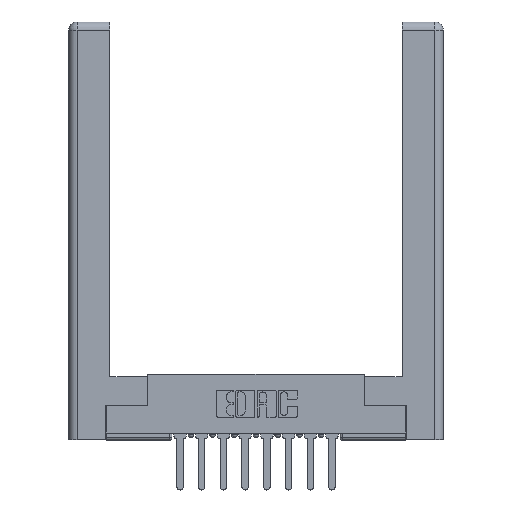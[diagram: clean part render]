
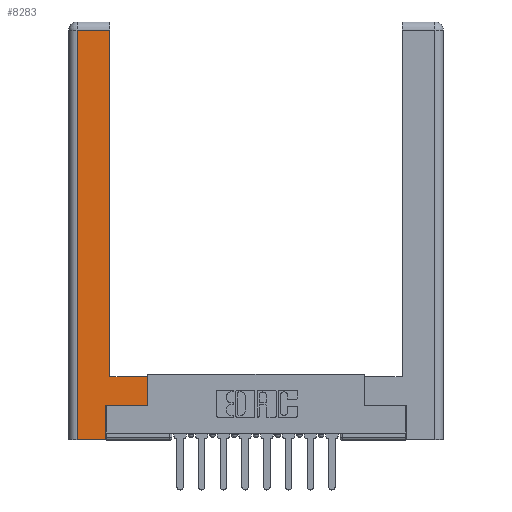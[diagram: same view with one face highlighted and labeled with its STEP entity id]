
A CAD part, top view. The second image highlights one B-rep face of the part: STEP entity #8283.
In plain terms, the highlighted planar face has unit normal (0, 0, 1).
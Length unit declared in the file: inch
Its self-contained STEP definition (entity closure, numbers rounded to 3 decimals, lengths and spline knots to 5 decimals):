
#43 = CARTESIAN_POINT ( 'NONE',  ( 0.295, 2.94, 0. ) ) ;
#262 = CARTESIAN_POINT ( 'NONE',  ( 0.0615, 2.94, 0. ) ) ;
#449 = CARTESIAN_POINT ( 'NONE',  ( 0.265, 0.245, 0. ) ) ;
#627 = VECTOR ( 'NONE', #13145, 39.37008 ) ;
#644 = AXIS2_PLACEMENT_3D ( 'NONE', #8451, #4155, #2939 ) ;
#757 = CARTESIAN_POINT ( 'NONE',  ( 0.565, 0.45, 0. ) ) ;
#957 = CARTESIAN_POINT ( 'NONE',  ( 0.295, 0.45, 0. ) ) ;
#1875 = EDGE_CURVE ( 'NONE', #13358, #9814, #12381, .T. ) ;
#2027 = ORIENTED_EDGE ( 'NONE', *, *, #13326, .T. ) ;
#2214 = VECTOR ( 'NONE', #12709, 39.37008 ) ;
#2616 = CARTESIAN_POINT ( 'NONE',  ( 0.565, 0.245, 0. ) ) ;
#2684 = LINE ( 'NONE', #2616, #5479 ) ;
#2905 = CARTESIAN_POINT ( 'NONE',  ( 0.0615, 0., 0. ) ) ;
#2939 = DIRECTION ( 'NONE',  ( -1., 0., 0. ) ) ;
#3006 = DIRECTION ( 'NONE',  ( 1., 0., 0. ) ) ;
#3062 = ORIENTED_EDGE ( 'NONE', *, *, #5730, .T. ) ;
#3267 = CARTESIAN_POINT ( 'NONE',  ( 0.265, 0., 0. ) ) ;
#3303 = CARTESIAN_POINT ( 'NONE',  ( 0.295, 3., 0. ) ) ;
#3328 = EDGE_CURVE ( 'NONE', #13282, #8489, #5622, .T. ) ;
#3491 = DIRECTION ( 'NONE',  ( 0., 1., 0. ) ) ;
#3493 = EDGE_CURVE ( 'NONE', #13676, #13358, #11300, .T. ) ;
#3692 = EDGE_CURVE ( 'NONE', #9814, #13282, #12748, .T. ) ;
#4155 = DIRECTION ( 'NONE',  ( 0., 0., -1. ) ) ;
#4262 = CARTESIAN_POINT ( 'NONE',  ( 0.565, 0.245, 0. ) ) ;
#5374 = ORIENTED_EDGE ( 'NONE', *, *, #3493, .T. ) ;
#5439 = VERTEX_POINT ( 'NONE', #8372 ) ;
#5479 = VECTOR ( 'NONE', #13273, 39.37008 ) ;
#5622 = LINE ( 'NONE', #449, #11181 ) ;
#5730 = EDGE_CURVE ( 'NONE', #5848, #5439, #12099, .T. ) ;
#5848 = VERTEX_POINT ( 'NONE', #4262 ) ;
#6094 = VECTOR ( 'NONE', #13320, 39.37008 ) ;
#6099 = EDGE_CURVE ( 'NONE', #8489, #5848, #2684, .T. ) ;
#7888 = CARTESIAN_POINT ( 'NONE',  ( 0.265, 0.245, 0. ) ) ;
#8128 = ORIENTED_EDGE ( 'NONE', *, *, #9293, .T. ) ;
#8283 = ADVANCED_FACE ( 'NONE', ( #13447 ), #10392, .F. ) ;
#8372 = CARTESIAN_POINT ( 'NONE',  ( 0.565, 0.45, 0. ) ) ;
#8451 = CARTESIAN_POINT ( 'NONE',  ( 0., 0., 0. ) ) ;
#8489 = VERTEX_POINT ( 'NONE', #7888 ) ;
#9293 = EDGE_CURVE ( 'NONE', #12340, #13676, #10488, .T. ) ;
#9304 = ORIENTED_EDGE ( 'NONE', *, *, #6099, .T. ) ;
#9694 = EDGE_LOOP ( 'NONE', ( #8128, #5374, #13259, #12666, #12852, #9304, #3062, #2027 ) ) ;
#9814 = VERTEX_POINT ( 'NONE', #11149 ) ;
#10054 = VECTOR ( 'NONE', #11330, 39.37008 ) ;
#10125 = VECTOR ( 'NONE', #13610, 39.37008 ) ;
#10392 = PLANE ( 'NONE',  #644 ) ;
#10423 = LINE ( 'NONE', #957, #10125 ) ;
#10488 = LINE ( 'NONE', #3303, #2214 ) ;
#11149 = CARTESIAN_POINT ( 'NONE',  ( 0.0615, 0., 0. ) ) ;
#11181 = VECTOR ( 'NONE', #3491, 39.37008 ) ;
#11300 = LINE ( 'NONE', #12135, #6094 ) ;
#11330 = DIRECTION ( 'NONE',  ( 0., -1., 0. ) ) ;
#12099 = LINE ( 'NONE', #757, #627 ) ;
#12135 = CARTESIAN_POINT ( 'NONE',  ( 0.0615, 2.94, 0. ) ) ;
#12215 = CARTESIAN_POINT ( 'NONE',  ( 0.295, 0.45, 0. ) ) ;
#12340 = VERTEX_POINT ( 'NONE', #12215 ) ;
#12381 = LINE ( 'NONE', #2905, #10054 ) ;
#12666 = ORIENTED_EDGE ( 'NONE', *, *, #3692, .T. ) ;
#12709 = DIRECTION ( 'NONE',  ( 0., 1., 0. ) ) ;
#12748 = LINE ( 'NONE', #3267, #13621 ) ;
#12850 = CARTESIAN_POINT ( 'NONE',  ( 0.265, 0., 0. ) ) ;
#12852 = ORIENTED_EDGE ( 'NONE', *, *, #3328, .T. ) ;
#13145 = DIRECTION ( 'NONE',  ( 0., 1., 0. ) ) ;
#13259 = ORIENTED_EDGE ( 'NONE', *, *, #1875, .T. ) ;
#13273 = DIRECTION ( 'NONE',  ( 1., 0., 0. ) ) ;
#13282 = VERTEX_POINT ( 'NONE', #12850 ) ;
#13320 = DIRECTION ( 'NONE',  ( -1., 0., 0. ) ) ;
#13326 = EDGE_CURVE ( 'NONE', #5439, #12340, #10423, .T. ) ;
#13358 = VERTEX_POINT ( 'NONE', #262 ) ;
#13447 = FACE_OUTER_BOUND ( 'NONE', #9694, .T. ) ;
#13610 = DIRECTION ( 'NONE',  ( -1., 0., 0. ) ) ;
#13621 = VECTOR ( 'NONE', #3006, 39.37008 ) ;
#13676 = VERTEX_POINT ( 'NONE', #43 ) ;
